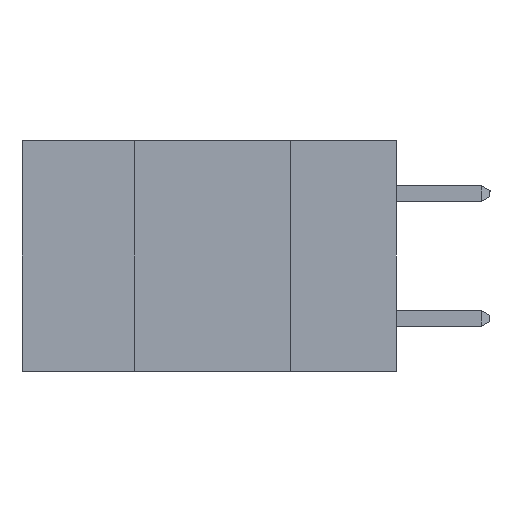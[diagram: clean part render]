
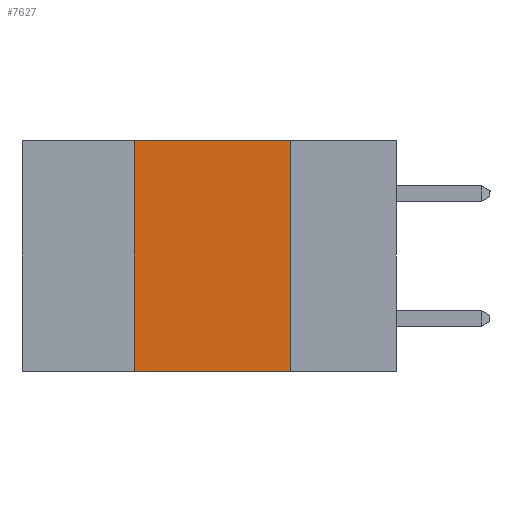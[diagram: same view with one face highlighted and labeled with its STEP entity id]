
A CAD part, left-side view. The second image highlights one B-rep face of the part: STEP entity #7627.
In plain terms, the highlighted planar face has unit normal (-1, 0, 0).
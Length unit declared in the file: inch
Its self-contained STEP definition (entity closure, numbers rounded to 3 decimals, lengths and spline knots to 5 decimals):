
#35 = VERTEX_POINT ( 'NONE', #10483 ) ;
#395 = VERTEX_POINT ( 'NONE', #10531 ) ;
#889 = EDGE_CURVE ( 'NONE', #7483, #35, #12343, .T. ) ;
#934 = LINE ( 'NONE', #8609, #1479 ) ;
#947 = CARTESIAN_POINT ( 'NONE',  ( 0., 0.6, -0.37 ) ) ;
#1322 = EDGE_CURVE ( 'NONE', #395, #35, #8907, .T. ) ;
#1479 = VECTOR ( 'NONE', #3960, 39.37008 ) ;
#1524 = ORIENTED_EDGE ( 'NONE', *, *, #5945, .F. ) ;
#1608 = ORIENTED_EDGE ( 'NONE', *, *, #889, .T. ) ;
#1845 = CARTESIAN_POINT ( 'NONE',  ( 0., 0.42, 0. ) ) ;
#2315 = VECTOR ( 'NONE', #8765, 39.37008 ) ;
#2572 = ORIENTED_EDGE ( 'NONE', *, *, #1322, .F. ) ;
#2949 = LINE ( 'NONE', #8343, #2315 ) ;
#3517 = FACE_OUTER_BOUND ( 'NONE', #5051, .T. ) ;
#3733 = DIRECTION ( 'NONE',  ( 0., -1., 0. ) ) ;
#3914 = VECTOR ( 'NONE', #4202, 39.37008 ) ;
#3960 = DIRECTION ( 'NONE',  ( 0., 0., 1. ) ) ;
#4202 = DIRECTION ( 'NONE',  ( 0., 0., -1. ) ) ;
#4402 = DIRECTION ( 'NONE',  ( 0., 0., -1. ) ) ;
#4838 = ORIENTED_EDGE ( 'NONE', *, *, #9535, .F. ) ;
#4972 = VERTEX_POINT ( 'NONE', #1845 ) ;
#5051 = EDGE_LOOP ( 'NONE', ( #2572, #4838, #1524, #1608 ) ) ;
#5945 = EDGE_CURVE ( 'NONE', #7483, #4972, #934, .T. ) ;
#6422 = PLANE ( 'NONE',  #9914 ) ;
#7411 = CARTESIAN_POINT ( 'NONE',  ( 0., 0.42, -0.37 ) ) ;
#7483 = VERTEX_POINT ( 'NONE', #7411 ) ;
#7627 = ADVANCED_FACE ( 'NONE', ( #3517 ), #6422, .F. ) ;
#8050 = VECTOR ( 'NONE', #3733, 39.37008 ) ;
#8343 = CARTESIAN_POINT ( 'NONE',  ( 0., 0.6, 0. ) ) ;
#8609 = CARTESIAN_POINT ( 'NONE',  ( 0., 0.42, -0.37 ) ) ;
#8765 = DIRECTION ( 'NONE',  ( 0., -1., 0. ) ) ;
#8907 = LINE ( 'NONE', #11804, #3914 ) ;
#9351 = DIRECTION ( 'NONE',  ( 1., 0., 0. ) ) ;
#9535 = EDGE_CURVE ( 'NONE', #4972, #395, #2949, .T. ) ;
#9914 = AXIS2_PLACEMENT_3D ( 'NONE', #12252, #9351, #4402 ) ;
#10483 = CARTESIAN_POINT ( 'NONE',  ( 0., 0.17, -0.37 ) ) ;
#10531 = CARTESIAN_POINT ( 'NONE',  ( 0., 0.17, 0. ) ) ;
#11804 = CARTESIAN_POINT ( 'NONE',  ( 0., 0.17, -0.37 ) ) ;
#12252 = CARTESIAN_POINT ( 'NONE',  ( 0., 0.6, 0. ) ) ;
#12343 = LINE ( 'NONE', #947, #8050 ) ;
